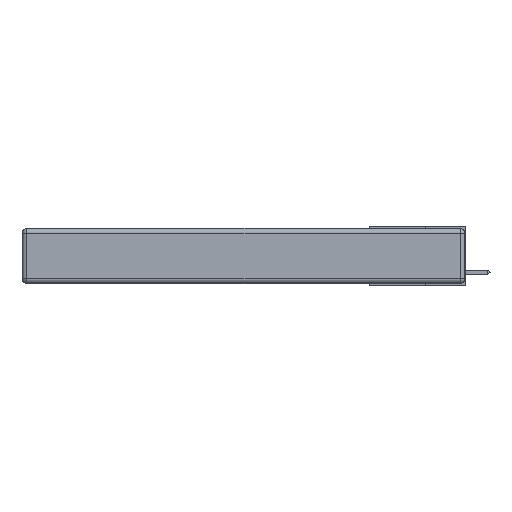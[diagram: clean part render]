
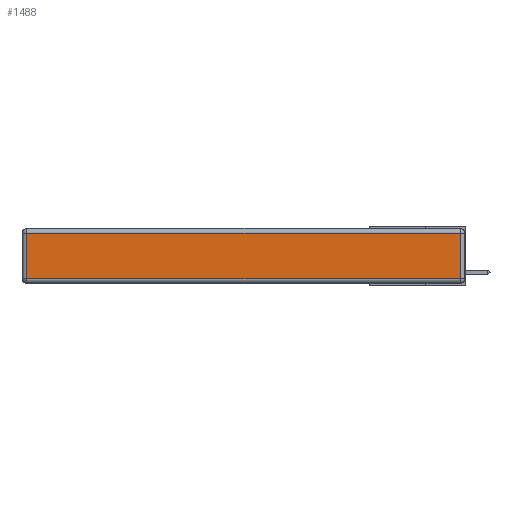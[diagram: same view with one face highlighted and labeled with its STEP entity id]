
A CAD part, left-side view. The second image highlights one B-rep face of the part: STEP entity #1488.
In plain terms, the highlighted planar face has unit normal (-1, 0, 0).
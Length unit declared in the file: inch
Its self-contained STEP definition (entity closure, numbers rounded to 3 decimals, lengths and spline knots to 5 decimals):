
#84 = VECTOR ( 'NONE', #4370, 39.37008 ) ;
#594 = AXIS2_PLACEMENT_3D ( 'NONE', #23307, #13408, #9521 ) ;
#623 = EDGE_CURVE ( 'NONE', #13661, #3575, #2795, .T. ) ;
#1488 = ADVANCED_FACE ( 'NONE', ( #21183 ), #23143, .T. ) ;
#1767 = CARTESIAN_POINT ( 'NONE',  ( 0., 2.72, -0.313 ) ) ;
#2066 = CARTESIAN_POINT ( 'NONE',  ( 0., 2.72, -0.343 ) ) ;
#2305 = DIRECTION ( 'NONE',  ( 0., -1., 0. ) ) ;
#2408 = CARTESIAN_POINT ( 'NONE',  ( 0., 0.03, -0.03 ) ) ;
#2795 = LINE ( 'NONE', #11368, #7446 ) ;
#3232 = CARTESIAN_POINT ( 'NONE',  ( 0., 2.72, -0.03 ) ) ;
#3411 = LINE ( 'NONE', #2066, #21232 ) ;
#3575 = VERTEX_POINT ( 'NONE', #3232 ) ;
#4370 = DIRECTION ( 'NONE',  ( 0., 0., 1. ) ) ;
#6769 = EDGE_CURVE ( 'NONE', #16157, #14193, #10206, .T. ) ;
#7446 = VECTOR ( 'NONE', #9663, 39.37008 ) ;
#9521 = DIRECTION ( 'NONE',  ( 0., 0., 1. ) ) ;
#9663 = DIRECTION ( 'NONE',  ( 0., 1., 0. ) ) ;
#10206 = LINE ( 'NONE', #22047, #18175 ) ;
#11368 = CARTESIAN_POINT ( 'NONE',  ( 0., 2.75, -0.03 ) ) ;
#13082 = CARTESIAN_POINT ( 'NONE',  ( 0., 0.03, -0.313 ) ) ;
#13189 = EDGE_CURVE ( 'NONE', #14193, #13661, #24327, .T. ) ;
#13408 = DIRECTION ( 'NONE',  ( -1., 0., 0. ) ) ;
#13661 = VERTEX_POINT ( 'NONE', #2408 ) ;
#14193 = VERTEX_POINT ( 'NONE', #13082 ) ;
#15883 = DIRECTION ( 'NONE',  ( 0., 0., -1. ) ) ;
#16157 = VERTEX_POINT ( 'NONE', #1767 ) ;
#16887 = EDGE_CURVE ( 'NONE', #3575, #16157, #3411, .T. ) ;
#17912 = EDGE_LOOP ( 'NONE', ( #17974, #22570, #20155, #22483 ) ) ;
#17974 = ORIENTED_EDGE ( 'NONE', *, *, #6769, .T. ) ;
#18175 = VECTOR ( 'NONE', #2305, 39.37008 ) ;
#20087 = CARTESIAN_POINT ( 'NONE',  ( 0., 0.03, -0.343 ) ) ;
#20155 = ORIENTED_EDGE ( 'NONE', *, *, #623, .T. ) ;
#21183 = FACE_OUTER_BOUND ( 'NONE', #17912, .T. ) ;
#21232 = VECTOR ( 'NONE', #15883, 39.37008 ) ;
#22047 = CARTESIAN_POINT ( 'NONE',  ( 0., 0., -0.313 ) ) ;
#22483 = ORIENTED_EDGE ( 'NONE', *, *, #16887, .T. ) ;
#22570 = ORIENTED_EDGE ( 'NONE', *, *, #13189, .T. ) ;
#23143 = PLANE ( 'NONE',  #594 ) ;
#23307 = CARTESIAN_POINT ( 'NONE',  ( 0., 0., -0.343 ) ) ;
#24327 = LINE ( 'NONE', #20087, #84 ) ;
